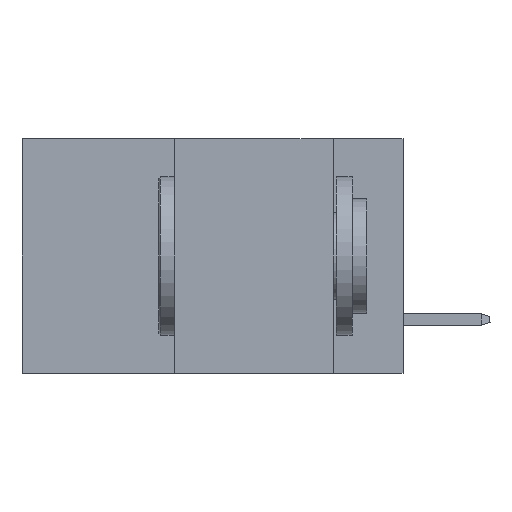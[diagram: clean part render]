
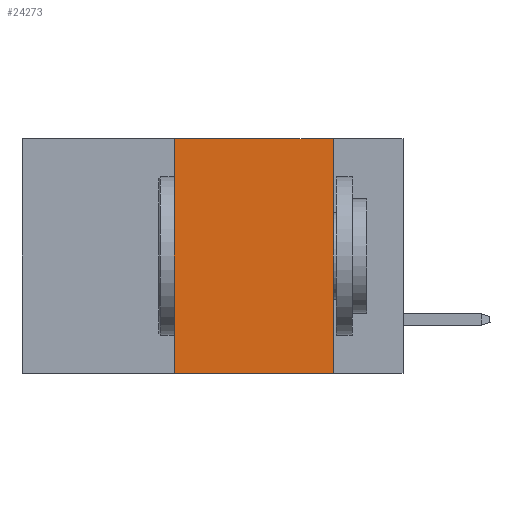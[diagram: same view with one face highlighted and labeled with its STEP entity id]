
A CAD part, left-side view. The second image highlights one B-rep face of the part: STEP entity #24273.
In plain terms, the highlighted planar face has unit normal (-1, 0, 0).
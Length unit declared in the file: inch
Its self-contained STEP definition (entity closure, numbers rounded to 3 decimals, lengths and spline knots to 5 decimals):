
#666 = EDGE_LOOP ( 'NONE', ( #7375, #34011, #23516, #19635 ) ) ;
#2794 = CARTESIAN_POINT ( 'NONE',  ( 0., 0.36, 0. ) ) ;
#3271 = VERTEX_POINT ( 'NONE', #13175 ) ;
#3610 = DIRECTION ( 'NONE',  ( 0., 0., -1. ) ) ;
#3736 = VECTOR ( 'NONE', #17290, 39.37008 ) ;
#4048 = EDGE_CURVE ( 'NONE', #23319, #3271, #30065, .T. ) ;
#5763 = VECTOR ( 'NONE', #26742, 39.37008 ) ;
#6376 = CARTESIAN_POINT ( 'NONE',  ( 0., 0.6, 0. ) ) ;
#7375 = ORIENTED_EDGE ( 'NONE', *, *, #10311, .F. ) ;
#8932 = VERTEX_POINT ( 'NONE', #32458 ) ;
#9508 = DIRECTION ( 'NONE',  ( 0., -1., 0. ) ) ;
#10311 = EDGE_CURVE ( 'NONE', #30107, #3271, #16705, .T. ) ;
#11073 = CARTESIAN_POINT ( 'NONE',  ( 0., 0.36, -0.37 ) ) ;
#13175 = CARTESIAN_POINT ( 'NONE',  ( 0., 0.11, -0.37 ) ) ;
#13385 = VECTOR ( 'NONE', #34569, 39.37008 ) ;
#13389 = CARTESIAN_POINT ( 'NONE',  ( 0., 0.6, -0.37 ) ) ;
#14539 = CARTESIAN_POINT ( 'NONE',  ( 0., 0.11, 0. ) ) ;
#14976 = LINE ( 'NONE', #2794, #5763 ) ;
#15224 = FACE_OUTER_BOUND ( 'NONE', #666, .T. ) ;
#16705 = LINE ( 'NONE', #14539, #3736 ) ;
#17290 = DIRECTION ( 'NONE',  ( 0., 0., -1. ) ) ;
#19635 = ORIENTED_EDGE ( 'NONE', *, *, #4048, .T. ) ;
#19778 = EDGE_CURVE ( 'NONE', #23319, #8932, #14976, .T. ) ;
#21324 = PLANE ( 'NONE',  #28882 ) ;
#22260 = CARTESIAN_POINT ( 'NONE',  ( 0., 0.11, 0. ) ) ;
#23319 = VERTEX_POINT ( 'NONE', #11073 ) ;
#23516 = ORIENTED_EDGE ( 'NONE', *, *, #19778, .F. ) ;
#24273 = ADVANCED_FACE ( 'NONE', ( #15224 ), #21324, .F. ) ;
#25377 = DIRECTION ( 'NONE',  ( 1., 0., 0. ) ) ;
#26742 = DIRECTION ( 'NONE',  ( 0., 0., 1. ) ) ;
#28882 = AXIS2_PLACEMENT_3D ( 'NONE', #6376, #25377, #3610 ) ;
#30065 = LINE ( 'NONE', #13389, #34503 ) ;
#30107 = VERTEX_POINT ( 'NONE', #22260 ) ;
#32458 = CARTESIAN_POINT ( 'NONE',  ( 0., 0.36, 0. ) ) ;
#34011 = ORIENTED_EDGE ( 'NONE', *, *, #36767, .F. ) ;
#34503 = VECTOR ( 'NONE', #9508, 39.37008 ) ;
#34569 = DIRECTION ( 'NONE',  ( 0., -1., 0. ) ) ;
#34737 = CARTESIAN_POINT ( 'NONE',  ( 0., 0.6, 0. ) ) ;
#36767 = EDGE_CURVE ( 'NONE', #8932, #30107, #37863, .T. ) ;
#37863 = LINE ( 'NONE', #34737, #13385 ) ;
